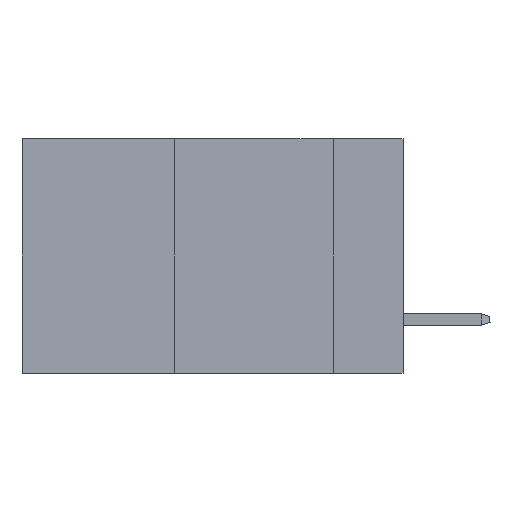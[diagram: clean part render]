
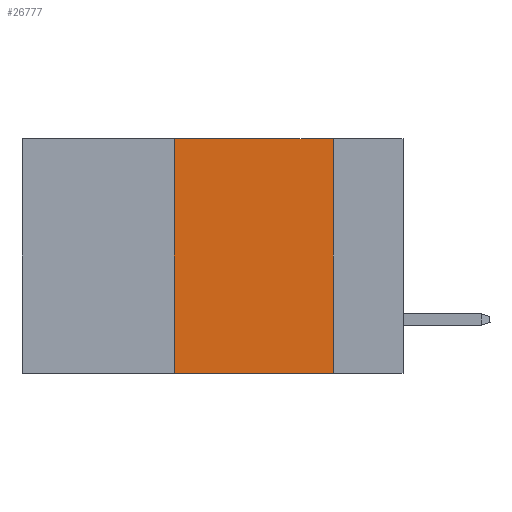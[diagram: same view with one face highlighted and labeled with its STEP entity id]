
A CAD part, left-side view. The second image highlights one B-rep face of the part: STEP entity #26777.
In plain terms, the highlighted planar face has unit normal (-1, 0, 0).
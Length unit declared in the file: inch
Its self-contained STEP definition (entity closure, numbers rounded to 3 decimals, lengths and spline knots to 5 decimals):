
#428 = CARTESIAN_POINT ( 'NONE',  ( 0., 0.11, 0. ) ) ;
#1457 = DIRECTION ( 'NONE',  ( 0., 0., 1. ) ) ;
#2938 = VERTEX_POINT ( 'NONE', #23401 ) ;
#2948 = DIRECTION ( 'NONE',  ( 0., 0., -1. ) ) ;
#3429 = AXIS2_PLACEMENT_3D ( 'NONE', #6430, #3953, #23359 ) ;
#3815 = CARTESIAN_POINT ( 'NONE',  ( 0., 0.36, -0.37 ) ) ;
#3825 = LINE ( 'NONE', #9798, #9637 ) ;
#3953 = DIRECTION ( 'NONE',  ( 1., 0., 0. ) ) ;
#6430 = CARTESIAN_POINT ( 'NONE',  ( 0., 0.6, 0. ) ) ;
#6555 = VERTEX_POINT ( 'NONE', #23231 ) ;
#7830 = VERTEX_POINT ( 'NONE', #428 ) ;
#8204 = LINE ( 'NONE', #8482, #19427 ) ;
#8482 = CARTESIAN_POINT ( 'NONE',  ( 0., 0.6, -0.37 ) ) ;
#9549 = ORIENTED_EDGE ( 'NONE', *, *, #12438, .F. ) ;
#9637 = VECTOR ( 'NONE', #1457, 39.37008 ) ;
#9745 = EDGE_LOOP ( 'NONE', ( #13092, #19930, #9549, #24929 ) ) ;
#9798 = CARTESIAN_POINT ( 'NONE',  ( 0., 0.36, 0. ) ) ;
#10253 = VERTEX_POINT ( 'NONE', #3815 ) ;
#10950 = LINE ( 'NONE', #17727, #24433 ) ;
#12438 = EDGE_CURVE ( 'NONE', #10253, #6555, #3825, .T. ) ;
#13092 = ORIENTED_EDGE ( 'NONE', *, *, #19790, .F. ) ;
#13451 = EDGE_CURVE ( 'NONE', #10253, #2938, #8204, .T. ) ;
#13494 = CARTESIAN_POINT ( 'NONE',  ( 0., 0.11, 0. ) ) ;
#14337 = PLANE ( 'NONE',  #3429 ) ;
#16936 = DIRECTION ( 'NONE',  ( 0., -1., 0. ) ) ;
#17727 = CARTESIAN_POINT ( 'NONE',  ( 0., 0.6, 0. ) ) ;
#19248 = EDGE_CURVE ( 'NONE', #6555, #7830, #10950, .T. ) ;
#19427 = VECTOR ( 'NONE', #16936, 39.37008 ) ;
#19590 = VECTOR ( 'NONE', #2948, 39.37008 ) ;
#19660 = DIRECTION ( 'NONE',  ( 0., -1., 0. ) ) ;
#19790 = EDGE_CURVE ( 'NONE', #7830, #2938, #26553, .T. ) ;
#19930 = ORIENTED_EDGE ( 'NONE', *, *, #19248, .F. ) ;
#22956 = FACE_OUTER_BOUND ( 'NONE', #9745, .T. ) ;
#23231 = CARTESIAN_POINT ( 'NONE',  ( 0., 0.36, 0. ) ) ;
#23359 = DIRECTION ( 'NONE',  ( 0., 0., -1. ) ) ;
#23401 = CARTESIAN_POINT ( 'NONE',  ( 0., 0.11, -0.37 ) ) ;
#24433 = VECTOR ( 'NONE', #19660, 39.37008 ) ;
#24929 = ORIENTED_EDGE ( 'NONE', *, *, #13451, .T. ) ;
#26553 = LINE ( 'NONE', #13494, #19590 ) ;
#26777 = ADVANCED_FACE ( 'NONE', ( #22956 ), #14337, .F. ) ;
